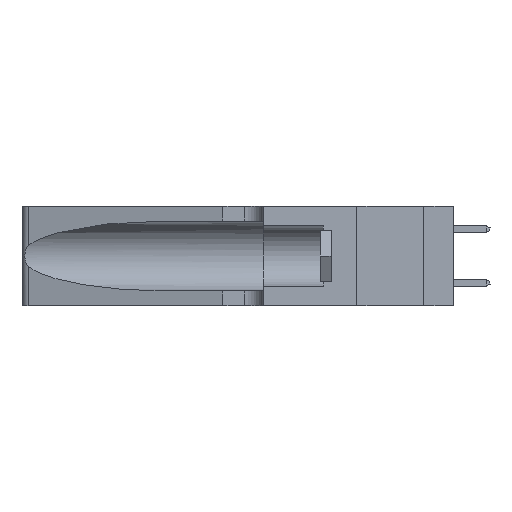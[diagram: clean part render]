
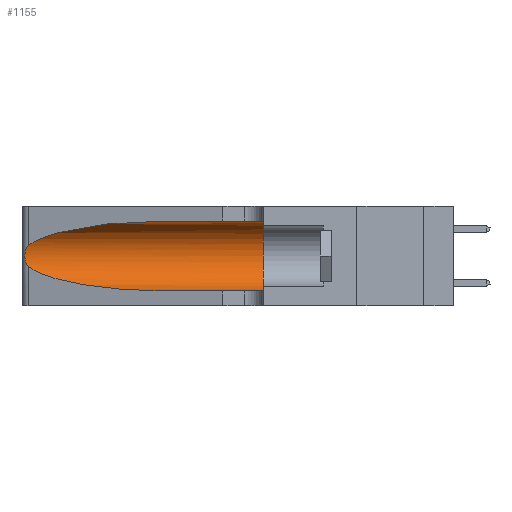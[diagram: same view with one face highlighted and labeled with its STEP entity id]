
A CAD part, left-side view. The second image highlights one B-rep face of the part: STEP entity #1155.
In plain terms, the highlighted cylindrical face has radius 3.308 mm (diameter 6.617 mm), a partial arc.
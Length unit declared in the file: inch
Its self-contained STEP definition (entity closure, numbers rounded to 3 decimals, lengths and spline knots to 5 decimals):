
#288 = LINE ( 'NONE', #31108, #27648 ) ;
#451 = CARTESIAN_POINT ( 'NONE',  ( 0.1305, 0.72297, 0.31525 ) ) ;
#1155 = ADVANCED_FACE ( 'NONE', ( #25757 ), #23468, .F. ) ;
#2027 = DIRECTION ( 'NONE',  ( 0., 0., -1. ) ) ;
#2119 = EDGE_CURVE ( 'NONE', #10349, #23280, #20781, .T. ) ;
#2344 = B_SPLINE_CURVE_WITH_KNOTS ( 'NONE', 3,
 ( #6868, #26276, #22174, #9707, #24306, #17321, #29396, #10000, #5321, #19803, #14877, #26880, #17415, #5126 ),
 .UNSPECIFIED., .F., .F.,
 ( 4, 2, 2, 2, 2, 2, 4 ),
 ( 0., 0.00027, 0.00053, 0.00107, 0.0016, 0.00187, 0.00214 ),
 .UNSPECIFIED. ) ;
#2859 = ORIENTED_EDGE ( 'NONE', *, *, #2119, .T. ) ;
#4268 = CARTESIAN_POINT ( 'NONE',  ( 0.1305, 1.61858, 0.185 ) ) ;
#4589 = LINE ( 'NONE', #4918, #6486 ) ;
#4608 = CARTESIAN_POINT ( 'NONE',  ( 0.25487, 1.22718, 0.22369 ) ) ;
#4918 = CARTESIAN_POINT ( 'NONE',  ( 0.1305, 1.61858, 0.31525 ) ) ;
#5126 = CARTESIAN_POINT ( 'NONE',  ( 0.25487, 1.22718, 0.14631 ) ) ;
#5321 = CARTESIAN_POINT ( 'NONE',  ( 0.26017, 1.23833, 0.17102 ) ) ;
#5323 = VERTEX_POINT ( 'NONE', #4608 ) ;
#6486 = VECTOR ( 'NONE', #7164, 39.37008 ) ;
#6576 = CARTESIAN_POINT ( 'NONE',  ( 0.2373, 1.15595, 0.08982 ) ) ;
#6836 = DIRECTION ( 'NONE',  ( 0., -1., 0. ) ) ;
#6868 = CARTESIAN_POINT ( 'NONE',  ( 0.25487, 1.22718, 0.22369 ) ) ;
#7164 = DIRECTION ( 'NONE',  ( 0., -1., 0. ) ) ;
#8507 = VERTEX_POINT ( 'NONE', #19575 ) ;
#8736 = ORIENTED_EDGE ( 'NONE', *, *, #25194, .F. ) ;
#9707 = CARTESIAN_POINT ( 'NONE',  ( 0.25787, 1.23484, 0.2124 ) ) ;
#10000 = CARTESIAN_POINT ( 'NONE',  ( 0.26075, 1.23896, 0.178 ) ) ;
#10349 = VERTEX_POINT ( 'NONE', #13795 ) ;
#11388 = VERTEX_POINT ( 'NONE', #451 ) ;
#13795 = CARTESIAN_POINT ( 'NONE',  ( 0.25487, 1.22718, 0.14631 ) ) ;
#14877 = CARTESIAN_POINT ( 'NONE',  ( 0.25789, 1.23486, 0.15765 ) ) ;
#15307 = AXIS2_PLACEMENT_3D ( 'NONE', #4268, #19099, #2027 ) ;
#15989 = DIRECTION ( 'NONE',  ( 0., 1., 0. ) ) ;
#16269 = EDGE_CURVE ( 'NONE', #11388, #5323, #21924, .T. ) ;
#16285 = CARTESIAN_POINT ( 'NONE',  ( 0.1305, 0.35, 0.31525 ) ) ;
#16383 = ORIENTED_EDGE ( 'NONE', *, *, #30800, .T. ) ;
#16619 = CARTESIAN_POINT ( 'NONE',  ( 0.25487, 1.22718, 0.14631 ) ) ;
#17321 = CARTESIAN_POINT ( 'NONE',  ( 0.26018, 1.23835, 0.19895 ) ) ;
#17415 = CARTESIAN_POINT ( 'NONE',  ( 0.25555, 1.22993, 0.14849 ) ) ;
#17952 = EDGE_CURVE ( 'NONE', #23280, #8507, #288, .T. ) ;
#19099 = DIRECTION ( 'NONE',  ( 0., -1., 0. ) ) ;
#19575 = CARTESIAN_POINT ( 'NONE',  ( 0.1305, 0.35, 0.05475 ) ) ;
#19803 = CARTESIAN_POINT ( 'NONE',  ( 0.25856, 1.23593, 0.16098 ) ) ;
#20781 =( BOUNDED_CURVE ( )  B_SPLINE_CURVE ( 3, ( #16619, #6576, #21039, #30611 ),
 .UNSPECIFIED., .F., .F. ) 
 B_SPLINE_CURVE_WITH_KNOTS ( ( 4, 4 ),
 ( 3.44316, 4.71239 ),
 .UNSPECIFIED. ) 
 CURVE ( )  GEOMETRIC_REPRESENTATION_ITEM ( )  RATIONAL_B_SPLINE_CURVE ( ( 1., 0.87, 0.87, 1. ) ) 
 REPRESENTATION_ITEM ( '' )  );
#21039 = CARTESIAN_POINT ( 'NONE',  ( 0.18966, 0.96281, 0.05475 ) ) ;
#21210 = VERTEX_POINT ( 'NONE', #16285 ) ;
#21575 = EDGE_LOOP ( 'NONE', ( #29231, #16383, #2859, #22945, #30675, #8736 ) ) ;
#21924 =( BOUNDED_CURVE ( )  B_SPLINE_CURVE ( 3, ( #23582, #28472, #25823, #28795 ),
 .UNSPECIFIED., .F., .T. ) 
 B_SPLINE_CURVE_WITH_KNOTS ( ( 4, 4 ),
 ( 1.5708, 2.84003 ),
 .UNSPECIFIED. ) 
 CURVE ( )  GEOMETRIC_REPRESENTATION_ITEM ( )  RATIONAL_B_SPLINE_CURVE ( ( 1., 0.87, 0.87, 1. ) ) 
 REPRESENTATION_ITEM ( '' )  );
#22075 = CIRCLE ( 'NONE', #22610, 0.13025 ) ;
#22174 = CARTESIAN_POINT ( 'NONE',  ( 0.25639, 1.23184, 0.21858 ) ) ;
#22610 = AXIS2_PLACEMENT_3D ( 'NONE', #30714, #15989, #30610 ) ;
#22945 = ORIENTED_EDGE ( 'NONE', *, *, #17952, .T. ) ;
#23280 = VERTEX_POINT ( 'NONE', #30882 ) ;
#23468 = CYLINDRICAL_SURFACE ( 'NONE', #15307, 0.13025 ) ;
#23582 = CARTESIAN_POINT ( 'NONE',  ( 0.1305, 0.72297, 0.31525 ) ) ;
#24306 = CARTESIAN_POINT ( 'NONE',  ( 0.25854, 1.2359, 0.20912 ) ) ;
#25194 = EDGE_CURVE ( 'NONE', #11388, #21210, #4589, .T. ) ;
#25757 = FACE_OUTER_BOUND ( 'NONE', #21575, .T. ) ;
#25823 = CARTESIAN_POINT ( 'NONE',  ( 0.2373, 1.15595, 0.28018 ) ) ;
#26276 = CARTESIAN_POINT ( 'NONE',  ( 0.25555, 1.22994, 0.2215 ) ) ;
#26880 = CARTESIAN_POINT ( 'NONE',  ( 0.25639, 1.23186, 0.15144 ) ) ;
#27648 = VECTOR ( 'NONE', #6836, 39.37008 ) ;
#28472 = CARTESIAN_POINT ( 'NONE',  ( 0.18966, 0.96281, 0.31525 ) ) ;
#28795 = CARTESIAN_POINT ( 'NONE',  ( 0.25487, 1.22718, 0.22369 ) ) ;
#29231 = ORIENTED_EDGE ( 'NONE', *, *, #16269, .T. ) ;
#29396 = CARTESIAN_POINT ( 'NONE',  ( 0.26075, 1.23896, 0.19203 ) ) ;
#30567 = EDGE_CURVE ( 'NONE', #21210, #8507, #22075, .T. ) ;
#30610 = DIRECTION ( 'NONE',  ( 0., 0., 1. ) ) ;
#30611 = CARTESIAN_POINT ( 'NONE',  ( 0.1305, 0.72297, 0.05475 ) ) ;
#30675 = ORIENTED_EDGE ( 'NONE', *, *, #30567, .F. ) ;
#30714 = CARTESIAN_POINT ( 'NONE',  ( 0.1305, 0.35, 0.185 ) ) ;
#30800 = EDGE_CURVE ( 'NONE', #5323, #10349, #2344, .T. ) ;
#30882 = CARTESIAN_POINT ( 'NONE',  ( 0.1305, 0.72297, 0.05475 ) ) ;
#31108 = CARTESIAN_POINT ( 'NONE',  ( 0.1305, 1.61858, 0.05475 ) ) ;
